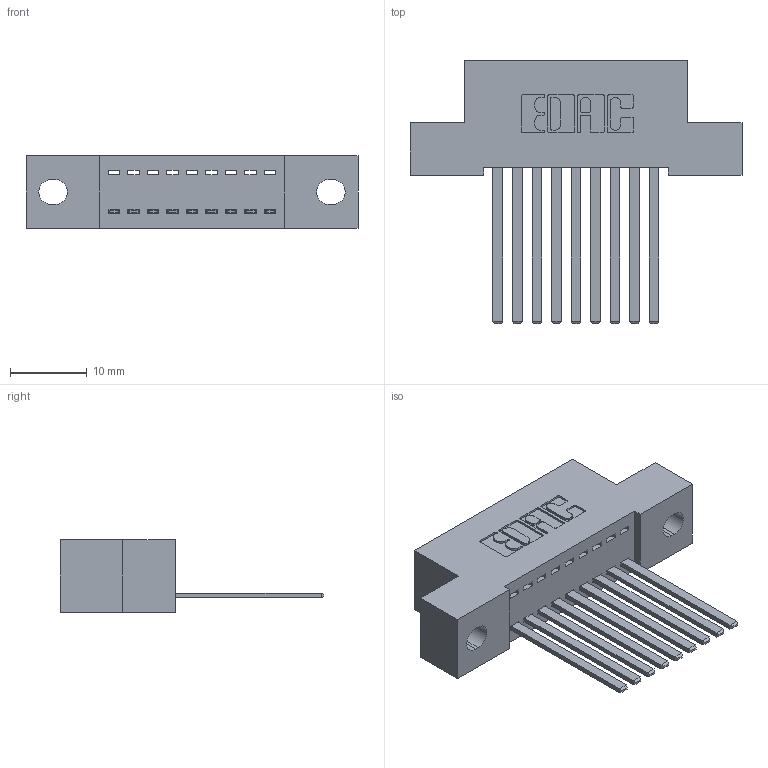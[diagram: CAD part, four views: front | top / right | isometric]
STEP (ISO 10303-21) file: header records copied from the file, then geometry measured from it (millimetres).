
FILE_DESCRIPTION (( 'STEP AP203' ), '1' );
FILE_NAME ('342-009-544-102.STEP', '2018-08-10T12:57:13', ( '' ), ( '' ), 'SwSTEP 2.0', 'SolidWorks 2016', '' );
FILE_SCHEMA (( 'CONFIG_CONTROL_DESIGN' ));
Length unit declared in the file: inch
Products named in the file (3): 342 Part_.128 Slot; 345-292-001_345-293-144; 342-009-544-102
Assembly tree (10 placements, depth 2):
  342-009-544-102
    342 Part_.128 Slot
    345-292-001_345-293-144  x9
Bounding box: 43.18 x 34.3 x 9.4 mm (x, y, z)
Volume: 3716.6 mm3; surface area: 4897.7 mm2
Topology: 10 solids, 10 shells, 582 faces, 1733 edges, 1142 vertices
Faces by surface type: plane 412, cylinder 170
Entity records: 9589 total; most frequent: CARTESIAN_POINT 1665, ORIENTED_EDGE 1610, DIRECTION 1467, EDGE_CURVE 805, VECTOR 681, LINE 681, VERTEX_POINT 534, AXIS2_PLACEMENT_3D 393
